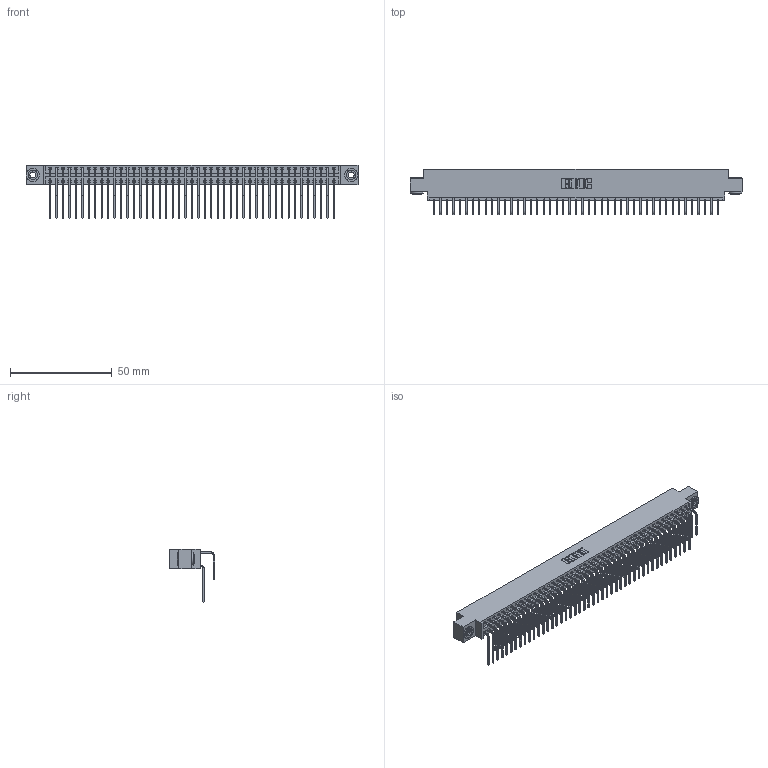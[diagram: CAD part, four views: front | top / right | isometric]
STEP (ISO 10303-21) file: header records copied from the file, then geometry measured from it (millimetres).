
FILE_DESCRIPTION (( 'STEP AP203' ), '1' );
FILE_NAME ('346-090-558-803.STEP', '2022-05-26T05:07:28', ( '' ), ( '' ), 'SwSTEP 2.0', 'SolidWorks 2020', '' );
FILE_SCHEMA (( 'CONFIG_CONTROL_DESIGN' ));
Length unit declared in the file: inch
Products named in the file (5): 345-292-001_558 Tail - 2; 345-250-002_345-250-002-102; 346 Part_0.170 Offset - 0.156 Dia-TH; 346-090-558-803; 345-292-001_558 559 Tail - 1
Assembly tree (93 placements, depth 2):
  346-090-558-803
    346 Part_0.170 Offset - 0.156 Dia-TH
    345-292-001_558 559 Tail - 1  x45
    345-292-001_558 Tail - 2  x45
    345-250-002_345-250-002-102  x2
Bounding box: 163.45 x 22.16 x 26.16 mm (x, y, z)
Volume: 16327.5 mm3; surface area: 25409.4 mm2
Topology: 93 solids, 93 shells, 5038 faces, 14943 edges, 9838 vertices
Faces by surface type: plane 3434, cylinder 1596, cone 8
Entity records: 31946 total; most frequent: CARTESIAN_POINT 5296, ORIENTED_EDGE 5170, DIRECTION 4719, EDGE_CURVE 2585, VECTOR 2209, LINE 2209, VERTEX_POINT 1718, AXIS2_PLACEMENT_3D 1255
